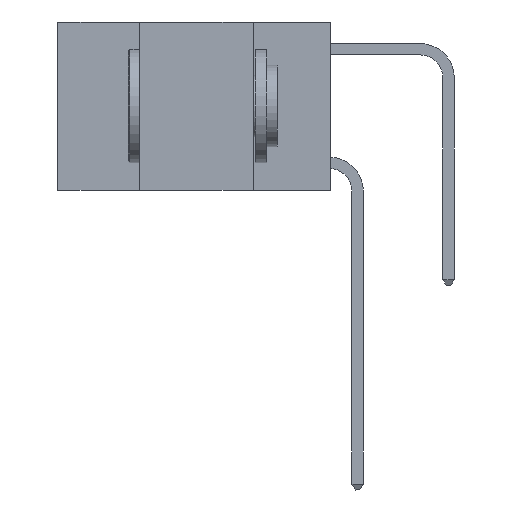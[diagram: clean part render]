
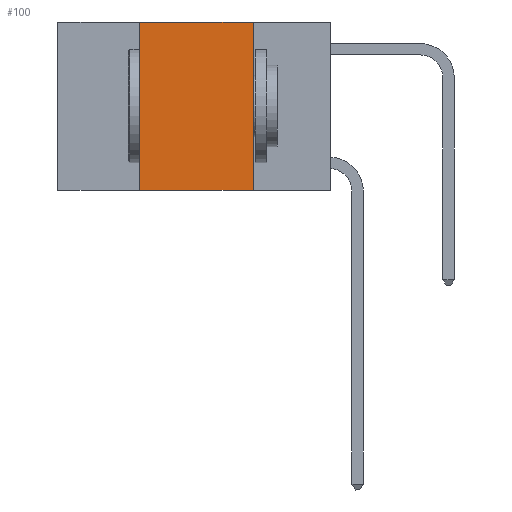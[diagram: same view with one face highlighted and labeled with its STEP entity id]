
A CAD part, left-side view. The second image highlights one B-rep face of the part: STEP entity #100.
In plain terms, the highlighted planar face has unit normal (-1, 0, 0).
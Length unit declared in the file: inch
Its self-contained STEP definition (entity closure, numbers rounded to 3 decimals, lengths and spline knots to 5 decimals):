
#73 = CARTESIAN_POINT ( 'NONE',  ( 0., 0.6, 0. ) ) ;
#100 = ADVANCED_FACE ( 'NONE', ( #1270 ), #1067, .F. ) ;
#150 = CARTESIAN_POINT ( 'NONE',  ( 0., 0.17, -0.37 ) ) ;
#342 = VERTEX_POINT ( 'NONE', #11125 ) ;
#550 = DIRECTION ( 'NONE',  ( 0., 0., 1. ) ) ;
#813 = DIRECTION ( 'NONE',  ( 1., 0., 0. ) ) ;
#897 = ORIENTED_EDGE ( 'NONE', *, *, #937, .T. ) ;
#937 = EDGE_CURVE ( 'NONE', #342, #8882, #9047, .T. ) ;
#1067 = PLANE ( 'NONE',  #9872 ) ;
#1270 = FACE_OUTER_BOUND ( 'NONE', #6348, .T. ) ;
#1831 = DIRECTION ( 'NONE',  ( 0., -1., 0. ) ) ;
#2182 = VERTEX_POINT ( 'NONE', #10950 ) ;
#2370 = LINE ( 'NONE', #10516, #7379 ) ;
#2408 = VECTOR ( 'NONE', #1831, 39.37008 ) ;
#5407 = ORIENTED_EDGE ( 'NONE', *, *, #8251, .F. ) ;
#5791 = VECTOR ( 'NONE', #550, 39.37008 ) ;
#5799 = CARTESIAN_POINT ( 'NONE',  ( 0., 0.17, 0. ) ) ;
#5864 = VECTOR ( 'NONE', #6707, 39.37008 ) ;
#6151 = LINE ( 'NONE', #5799, #5864 ) ;
#6348 = EDGE_LOOP ( 'NONE', ( #7490, #5407, #7782, #897 ) ) ;
#6707 = DIRECTION ( 'NONE',  ( 0., 0., -1. ) ) ;
#7379 = VECTOR ( 'NONE', #11390, 39.37008 ) ;
#7444 = CARTESIAN_POINT ( 'NONE',  ( 0., 0.42, 0. ) ) ;
#7490 = ORIENTED_EDGE ( 'NONE', *, *, #8121, .F. ) ;
#7574 = DIRECTION ( 'NONE',  ( 0., 0., -1. ) ) ;
#7782 = ORIENTED_EDGE ( 'NONE', *, *, #11147, .F. ) ;
#8121 = EDGE_CURVE ( 'NONE', #2182, #8882, #6151, .T. ) ;
#8251 = EDGE_CURVE ( 'NONE', #8546, #2182, #2370, .T. ) ;
#8546 = VERTEX_POINT ( 'NONE', #7444 ) ;
#8882 = VERTEX_POINT ( 'NONE', #150 ) ;
#9047 = LINE ( 'NONE', #9511, #2408 ) ;
#9511 = CARTESIAN_POINT ( 'NONE',  ( 0., 0.6, -0.37 ) ) ;
#9872 = AXIS2_PLACEMENT_3D ( 'NONE', #73, #813, #7574 ) ;
#10516 = CARTESIAN_POINT ( 'NONE',  ( 0., 0.6, 0. ) ) ;
#10942 = LINE ( 'NONE', #11386, #5791 ) ;
#10950 = CARTESIAN_POINT ( 'NONE',  ( 0., 0.17, 0. ) ) ;
#11125 = CARTESIAN_POINT ( 'NONE',  ( 0., 0.42, -0.37 ) ) ;
#11147 = EDGE_CURVE ( 'NONE', #342, #8546, #10942, .T. ) ;
#11386 = CARTESIAN_POINT ( 'NONE',  ( 0., 0.42, 0. ) ) ;
#11390 = DIRECTION ( 'NONE',  ( 0., -1., 0. ) ) ;
